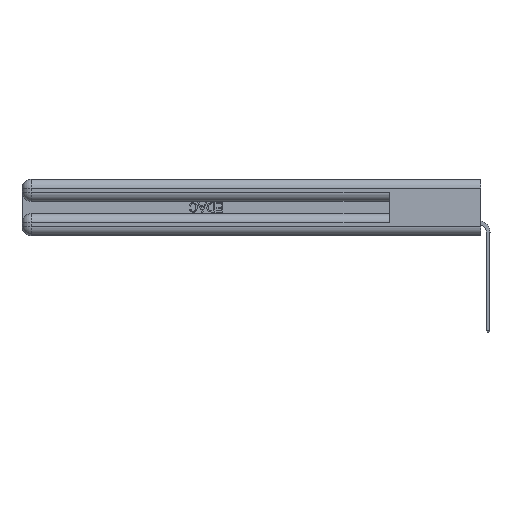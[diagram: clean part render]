
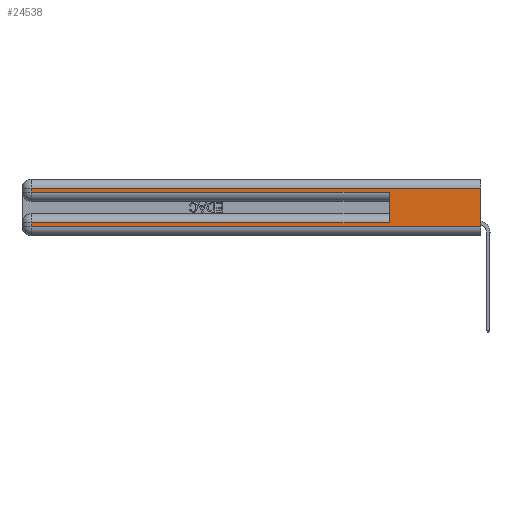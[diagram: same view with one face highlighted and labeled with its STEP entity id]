
A CAD part, left-side view. The second image highlights one B-rep face of the part: STEP entity #24538.
In plain terms, the highlighted planar face has unit normal (-1, 0, 0).
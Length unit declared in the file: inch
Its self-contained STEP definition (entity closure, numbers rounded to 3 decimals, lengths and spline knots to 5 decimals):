
#92 = VERTEX_POINT ( 'NONE', #19213 ) ;
#465 = EDGE_CURVE ( 'NONE', #29122, #13235, #37694, .T. ) ;
#500 = CARTESIAN_POINT ( 'NONE',  ( 0., 2.94, 0.31 ) ) ;
#676 = VERTEX_POINT ( 'NONE', #13170 ) ;
#1007 = DIRECTION ( 'NONE',  ( 0., 1., 0. ) ) ;
#1644 = CARTESIAN_POINT ( 'NONE',  ( 0., 2.94, 0.37 ) ) ;
#2152 = CARTESIAN_POINT ( 'NONE',  ( 0., 0.6, 0.285 ) ) ;
#2528 = PLANE ( 'NONE',  #4025 ) ;
#3549 = LINE ( 'NONE', #24932, #4041 ) ;
#3966 = VERTEX_POINT ( 'NONE', #24020 ) ;
#4025 = AXIS2_PLACEMENT_3D ( 'NONE', #5539, #31871, #35164 ) ;
#4041 = VECTOR ( 'NONE', #23486, 39.37008 ) ;
#4793 = DIRECTION ( 'NONE',  ( 0., 0., -1. ) ) ;
#5539 = CARTESIAN_POINT ( 'NONE',  ( 0., 0., 0.37 ) ) ;
#5938 = VECTOR ( 'NONE', #27902, 39.37008 ) ;
#6240 = EDGE_LOOP ( 'NONE', ( #18211, #6937, #38785, #30627, #21511, #24529, #42082, #15879 ) ) ;
#6937 = ORIENTED_EDGE ( 'NONE', *, *, #11007, .T. ) ;
#7730 = CARTESIAN_POINT ( 'NONE',  ( 0., 2.94, 0.06 ) ) ;
#8735 = VECTOR ( 'NONE', #4793, 39.37008 ) ;
#9067 = DIRECTION ( 'NONE',  ( 0., -1., 0. ) ) ;
#10293 = EDGE_CURVE ( 'NONE', #37208, #3966, #18458, .T. ) ;
#11007 = EDGE_CURVE ( 'NONE', #92, #24139, #3549, .T. ) ;
#11077 = VECTOR ( 'NONE', #26643, 39.37008 ) ;
#12804 = EDGE_CURVE ( 'NONE', #3966, #28150, #32060, .T. ) ;
#13170 = CARTESIAN_POINT ( 'NONE',  ( 0., 0., 0.06 ) ) ;
#13235 = VERTEX_POINT ( 'NONE', #2152 ) ;
#13646 = CARTESIAN_POINT ( 'NONE',  ( 0., 0., 0.37 ) ) ;
#13669 = VECTOR ( 'NONE', #34341, 39.37008 ) ;
#15879 = ORIENTED_EDGE ( 'NONE', *, *, #16224, .T. ) ;
#16224 = EDGE_CURVE ( 'NONE', #28150, #676, #39577, .T. ) ;
#17621 = EDGE_CURVE ( 'NONE', #24139, #29122, #29727, .T. ) ;
#18211 = ORIENTED_EDGE ( 'NONE', *, *, #27360, .F. ) ;
#18458 = LINE ( 'NONE', #30739, #35887 ) ;
#18527 = CARTESIAN_POINT ( 'NONE',  ( 0., 0., 0.285 ) ) ;
#19213 = CARTESIAN_POINT ( 'NONE',  ( 0., 0., 0.31 ) ) ;
#21511 = ORIENTED_EDGE ( 'NONE', *, *, #23356, .F. ) ;
#22374 = LINE ( 'NONE', #28023, #13669 ) ;
#23311 = VECTOR ( 'NONE', #41290, 39.37008 ) ;
#23356 = EDGE_CURVE ( 'NONE', #37208, #13235, #22374, .T. ) ;
#23486 = DIRECTION ( 'NONE',  ( 0., 1., 0. ) ) ;
#23663 = CARTESIAN_POINT ( 'NONE',  ( 0., 2.94, 0.285 ) ) ;
#24020 = CARTESIAN_POINT ( 'NONE',  ( 0., 2.94, 0.085 ) ) ;
#24139 = VERTEX_POINT ( 'NONE', #500 ) ;
#24529 = ORIENTED_EDGE ( 'NONE', *, *, #10293, .T. ) ;
#24538 = ADVANCED_FACE ( 'NONE', ( #29402 ), #2528, .F. ) ;
#24932 = CARTESIAN_POINT ( 'NONE',  ( 0., 0., 0.31 ) ) ;
#26643 = DIRECTION ( 'NONE',  ( 0., 0., -1. ) ) ;
#27360 = EDGE_CURVE ( 'NONE', #92, #676, #31004, .T. ) ;
#27366 = CARTESIAN_POINT ( 'NONE',  ( 0., 0., 0.06 ) ) ;
#27902 = DIRECTION ( 'NONE',  ( 0., 0., -1. ) ) ;
#28023 = CARTESIAN_POINT ( 'NONE',  ( 0., 0.6, 0.145 ) ) ;
#28150 = VERTEX_POINT ( 'NONE', #7730 ) ;
#29122 = VERTEX_POINT ( 'NONE', #23663 ) ;
#29402 = FACE_OUTER_BOUND ( 'NONE', #6240, .T. ) ;
#29727 = LINE ( 'NONE', #1644, #8735 ) ;
#30270 = CARTESIAN_POINT ( 'NONE',  ( 0., 0.6, 0.085 ) ) ;
#30627 = ORIENTED_EDGE ( 'NONE', *, *, #465, .T. ) ;
#30739 = CARTESIAN_POINT ( 'NONE',  ( 0., 0., 0.085 ) ) ;
#31004 = LINE ( 'NONE', #13646, #11077 ) ;
#31871 = DIRECTION ( 'NONE',  ( 1., 0., 0. ) ) ;
#32060 = LINE ( 'NONE', #34673, #5938 ) ;
#34341 = DIRECTION ( 'NONE',  ( 0., 0., 1. ) ) ;
#34415 = VECTOR ( 'NONE', #9067, 39.37008 ) ;
#34673 = CARTESIAN_POINT ( 'NONE',  ( 0., 2.94, 0.37 ) ) ;
#35164 = DIRECTION ( 'NONE',  ( 0., 0., -1. ) ) ;
#35887 = VECTOR ( 'NONE', #1007, 39.37008 ) ;
#37208 = VERTEX_POINT ( 'NONE', #30270 ) ;
#37694 = LINE ( 'NONE', #18527, #23311 ) ;
#38785 = ORIENTED_EDGE ( 'NONE', *, *, #17621, .T. ) ;
#39577 = LINE ( 'NONE', #27366, #34415 ) ;
#41290 = DIRECTION ( 'NONE',  ( 0., -1., 0. ) ) ;
#42082 = ORIENTED_EDGE ( 'NONE', *, *, #12804, .T. ) ;
